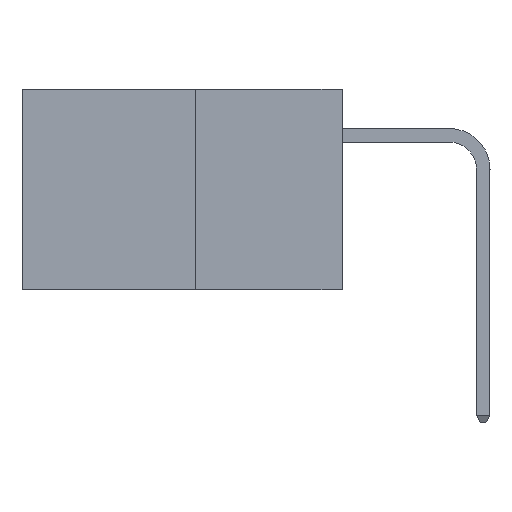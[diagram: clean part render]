
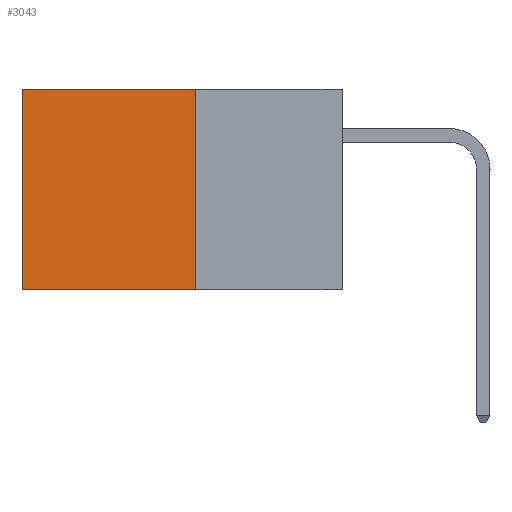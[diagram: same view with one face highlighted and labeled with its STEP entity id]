
A CAD part, left-side view. The second image highlights one B-rep face of the part: STEP entity #3043.
In plain terms, the highlighted planar face has unit normal (-1, 0, 0).
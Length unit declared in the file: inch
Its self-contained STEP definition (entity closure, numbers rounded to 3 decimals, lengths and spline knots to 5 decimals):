
#339 = FACE_OUTER_BOUND ( 'NONE', #436, .T. ) ;
#436 = EDGE_LOOP ( 'NONE', ( #7553, #7506, #7568, #7539 ) ) ;
#1063 = EDGE_CURVE ( 'NONE', #5404, #3522, #7767, .T. ) ;
#1603 = EDGE_CURVE ( 'NONE', #3522, #2550, #6898, .T. ) ;
#1927 = EDGE_CURVE ( 'NONE', #2064, #2550, #5224, .T. ) ;
#2000 = VECTOR ( 'NONE', #2617, 39.37008 ) ;
#2064 = VERTEX_POINT ( 'NONE', #4985 ) ;
#2077 = CARTESIAN_POINT ( 'NONE',  ( 0.277, 0.27, -0.37 ) ) ;
#2227 = EDGE_CURVE ( 'NONE', #5404, #2064, #7415, .T. ) ;
#2310 = CARTESIAN_POINT ( 'NONE',  ( 0.277, 0.27, 0. ) ) ;
#2461 = CARTESIAN_POINT ( 'NONE',  ( 0.277, 0.27, 0. ) ) ;
#2550 = VERTEX_POINT ( 'NONE', #3285 ) ;
#2612 = CARTESIAN_POINT ( 'NONE',  ( 0.277, 0.59, -0.37 ) ) ;
#2617 = DIRECTION ( 'NONE',  ( 0., 0., -1. ) ) ;
#2855 = DIRECTION ( 'NONE',  ( 0., 0., -1. ) ) ;
#2873 = VECTOR ( 'NONE', #6523, 39.37008 ) ;
#3043 = ADVANCED_FACE ( 'NONE', ( #339 ), #4684, .F. ) ;
#3285 = CARTESIAN_POINT ( 'NONE',  ( 0.277, 0.59, -0.37 ) ) ;
#3432 = CARTESIAN_POINT ( 'NONE',  ( 0.277, 0.27, -0.37 ) ) ;
#3522 = VERTEX_POINT ( 'NONE', #5013 ) ;
#3953 = DIRECTION ( 'NONE',  ( 1., 0., 0. ) ) ;
#4354 = DIRECTION ( 'NONE',  ( 0., 1., 0. ) ) ;
#4380 = DIRECTION ( 'NONE',  ( 0., 1., 0. ) ) ;
#4684 = PLANE ( 'NONE',  #5228 ) ;
#4985 = CARTESIAN_POINT ( 'NONE',  ( 0.277, 0.27, -0.37 ) ) ;
#5013 = CARTESIAN_POINT ( 'NONE',  ( 0.277, 0.59, 0. ) ) ;
#5224 = LINE ( 'NONE', #3432, #6488 ) ;
#5228 = AXIS2_PLACEMENT_3D ( 'NONE', #7127, #3953, #2855 ) ;
#5404 = VERTEX_POINT ( 'NONE', #2310 ) ;
#6488 = VECTOR ( 'NONE', #4380, 39.37008 ) ;
#6523 = DIRECTION ( 'NONE',  ( 0., 0., -1. ) ) ;
#6592 = VECTOR ( 'NONE', #4354, 39.37008 ) ;
#6898 = LINE ( 'NONE', #2612, #2000 ) ;
#7127 = CARTESIAN_POINT ( 'NONE',  ( 0.277, 0.27, -0.37 ) ) ;
#7415 = LINE ( 'NONE', #2077, #2873 ) ;
#7506 = ORIENTED_EDGE ( 'NONE', *, *, #1927, .F. ) ;
#7539 = ORIENTED_EDGE ( 'NONE', *, *, #1063, .T. ) ;
#7553 = ORIENTED_EDGE ( 'NONE', *, *, #1603, .T. ) ;
#7568 = ORIENTED_EDGE ( 'NONE', *, *, #2227, .F. ) ;
#7767 = LINE ( 'NONE', #2461, #6592 ) ;
